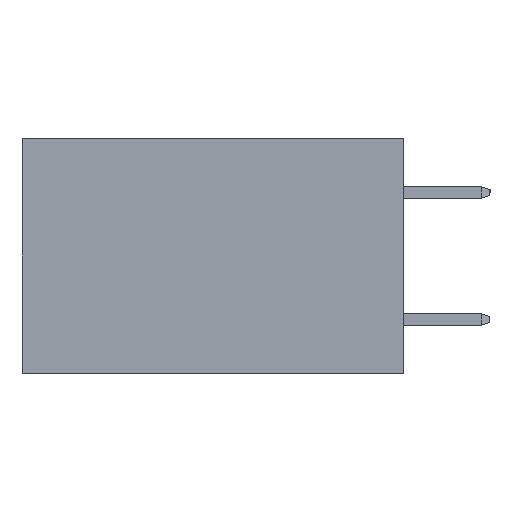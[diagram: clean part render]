
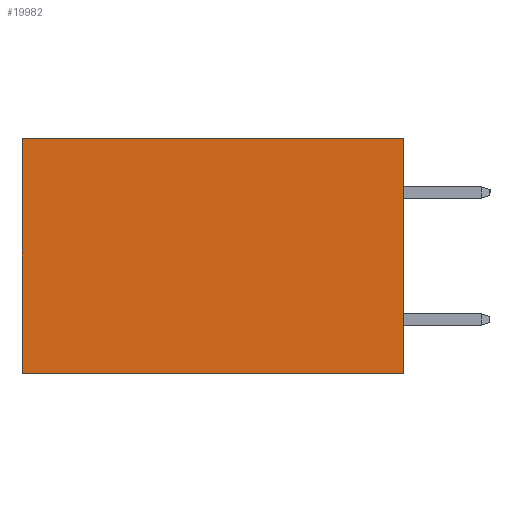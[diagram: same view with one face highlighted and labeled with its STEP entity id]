
A CAD part, left-side view. The second image highlights one B-rep face of the part: STEP entity #19982.
In plain terms, the highlighted planar face has unit normal (-1, 0, 0).
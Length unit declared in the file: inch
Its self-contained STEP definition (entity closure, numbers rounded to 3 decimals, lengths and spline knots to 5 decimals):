
#675 = LINE ( 'NONE', #16078, #31856 ) ;
#3010 = DIRECTION ( 'NONE',  ( 0., 0., -1. ) ) ;
#3257 = ORIENTED_EDGE ( 'NONE', *, *, #24018, .F. ) ;
#3309 = EDGE_CURVE ( 'NONE', #16152, #27749, #675, .T. ) ;
#5049 = CARTESIAN_POINT ( 'NONE',  ( 0.2875, 0.6, 0. ) ) ;
#5167 = VECTOR ( 'NONE', #16065, 39.37008 ) ;
#6057 = CARTESIAN_POINT ( 'NONE',  ( 0.2875, 0.6, 0. ) ) ;
#6428 = AXIS2_PLACEMENT_3D ( 'NONE', #17492, #28182, #15295 ) ;
#7227 = VECTOR ( 'NONE', #3010, 39.37008 ) ;
#7674 = FACE_OUTER_BOUND ( 'NONE', #13821, .T. ) ;
#7839 = CARTESIAN_POINT ( 'NONE',  ( 0.2875, 0., 0. ) ) ;
#9684 = ORIENTED_EDGE ( 'NONE', *, *, #14313, .T. ) ;
#10926 = VERTEX_POINT ( 'NONE', #5049 ) ;
#12149 = CARTESIAN_POINT ( 'NONE',  ( 0.2875, 0., -0.37 ) ) ;
#13155 = VECTOR ( 'NONE', #32627, 39.37008 ) ;
#13821 = EDGE_LOOP ( 'NONE', ( #13920, #3257, #27143, #9684 ) ) ;
#13920 = ORIENTED_EDGE ( 'NONE', *, *, #24307, .T. ) ;
#14313 = EDGE_CURVE ( 'NONE', #16152, #10926, #23700, .T. ) ;
#15190 = CARTESIAN_POINT ( 'NONE',  ( 0.2875, 0., -0.37 ) ) ;
#15295 = DIRECTION ( 'NONE',  ( 0., 0., -1. ) ) ;
#16065 = DIRECTION ( 'NONE',  ( 0., 1., 0. ) ) ;
#16078 = CARTESIAN_POINT ( 'NONE',  ( 0.2875, 0., 0. ) ) ;
#16152 = VERTEX_POINT ( 'NONE', #7839 ) ;
#16718 = LINE ( 'NONE', #6057, #7227 ) ;
#17278 = CARTESIAN_POINT ( 'NONE',  ( 0.2875, 0.6, -0.37 ) ) ;
#17492 = CARTESIAN_POINT ( 'NONE',  ( 0.2875, 0., 0. ) ) ;
#17552 = LINE ( 'NONE', #12149, #13155 ) ;
#18101 = CARTESIAN_POINT ( 'NONE',  ( 0.2875, 0., 0. ) ) ;
#19982 = ADVANCED_FACE ( 'NONE', ( #7674 ), #22917, .F. ) ;
#22917 = PLANE ( 'NONE',  #6428 ) ;
#23541 = DIRECTION ( 'NONE',  ( 0., 0., -1. ) ) ;
#23619 = VERTEX_POINT ( 'NONE', #17278 ) ;
#23700 = LINE ( 'NONE', #18101, #5167 ) ;
#24018 = EDGE_CURVE ( 'NONE', #27749, #23619, #17552, .T. ) ;
#24307 = EDGE_CURVE ( 'NONE', #10926, #23619, #16718, .T. ) ;
#27143 = ORIENTED_EDGE ( 'NONE', *, *, #3309, .F. ) ;
#27749 = VERTEX_POINT ( 'NONE', #15190 ) ;
#28182 = DIRECTION ( 'NONE',  ( 1., 0., 0. ) ) ;
#31856 = VECTOR ( 'NONE', #23541, 39.37008 ) ;
#32627 = DIRECTION ( 'NONE',  ( 0., 1., 0. ) ) ;
